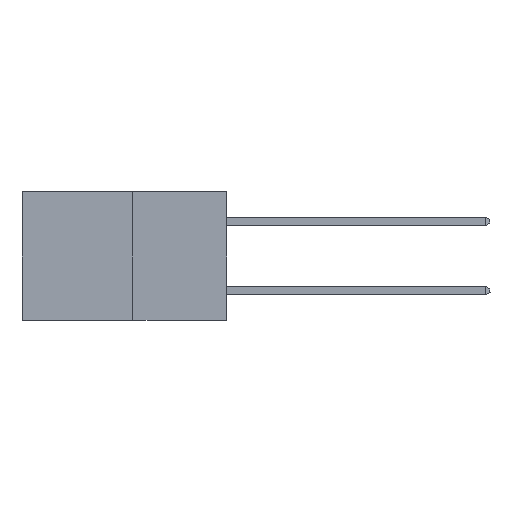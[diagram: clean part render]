
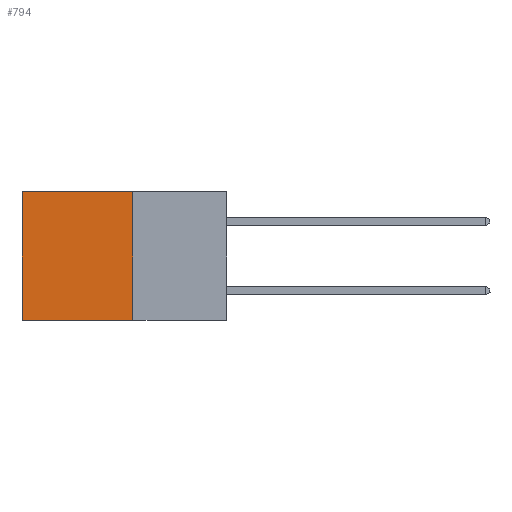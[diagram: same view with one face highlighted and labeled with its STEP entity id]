
A CAD part, left-side view. The second image highlights one B-rep face of the part: STEP entity #794.
In plain terms, the highlighted planar face has unit normal (-1, 0, 0).
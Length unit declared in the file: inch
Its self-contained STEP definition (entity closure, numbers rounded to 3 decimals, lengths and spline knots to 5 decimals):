
#794 = ADVANCED_FACE ( 'NONE', ( #16569 ), #21081, .F. ) ;
#3560 = CARTESIAN_POINT ( 'NONE',  ( 0.277, 0.27, 0. ) ) ;
#3947 = CARTESIAN_POINT ( 'NONE',  ( 0.277, 0.59, -0.37 ) ) ;
#4394 = EDGE_CURVE ( 'NONE', #24834, #8620, #6015, .T. ) ;
#4659 = DIRECTION ( 'NONE',  ( 1., 0., 0. ) ) ;
#5328 = VECTOR ( 'NONE', #27437, 39.37008 ) ;
#6015 = LINE ( 'NONE', #27498, #5328 ) ;
#6527 = CARTESIAN_POINT ( 'NONE',  ( 0.277, 0.27, -0.37 ) ) ;
#8620 = VERTEX_POINT ( 'NONE', #3947 ) ;
#8664 = DIRECTION ( 'NONE',  ( 0., 0., -1. ) ) ;
#8824 = EDGE_CURVE ( 'NONE', #20589, #24834, #24039, .T. ) ;
#9426 = CARTESIAN_POINT ( 'NONE',  ( 0.277, 0.59, -0.37 ) ) ;
#11299 = ORIENTED_EDGE ( 'NONE', *, *, #4394, .F. ) ;
#11416 = VECTOR ( 'NONE', #13048, 39.37008 ) ;
#12154 = EDGE_CURVE ( 'NONE', #25219, #8620, #25153, .T. ) ;
#12515 = CARTESIAN_POINT ( 'NONE',  ( 0.277, 0.59, 0. ) ) ;
#12981 = ORIENTED_EDGE ( 'NONE', *, *, #22750, .T. ) ;
#13013 = CARTESIAN_POINT ( 'NONE',  ( 0.277, 0.27, -0.37 ) ) ;
#13027 = DIRECTION ( 'NONE',  ( 0., 1., 0. ) ) ;
#13048 = DIRECTION ( 'NONE',  ( 0., 0., -1. ) ) ;
#15473 = LINE ( 'NONE', #17561, #28705 ) ;
#15789 = CARTESIAN_POINT ( 'NONE',  ( 0.277, 0.27, -0.37 ) ) ;
#16569 = FACE_OUTER_BOUND ( 'NONE', #19549, .T. ) ;
#17561 = CARTESIAN_POINT ( 'NONE',  ( 0.277, 0.27, 0. ) ) ;
#19256 = VECTOR ( 'NONE', #22971, 39.37008 ) ;
#19549 = EDGE_LOOP ( 'NONE', ( #25642, #11299, #28095, #12981 ) ) ;
#20589 = VERTEX_POINT ( 'NONE', #3560 ) ;
#21081 = PLANE ( 'NONE',  #27432 ) ;
#22750 = EDGE_CURVE ( 'NONE', #20589, #25219, #15473, .T. ) ;
#22971 = DIRECTION ( 'NONE',  ( 0., 0., -1. ) ) ;
#24039 = LINE ( 'NONE', #13013, #11416 ) ;
#24834 = VERTEX_POINT ( 'NONE', #15789 ) ;
#25153 = LINE ( 'NONE', #9426, #19256 ) ;
#25219 = VERTEX_POINT ( 'NONE', #12515 ) ;
#25642 = ORIENTED_EDGE ( 'NONE', *, *, #12154, .T. ) ;
#27432 = AXIS2_PLACEMENT_3D ( 'NONE', #6527, #4659, #8664 ) ;
#27437 = DIRECTION ( 'NONE',  ( 0., 1., 0. ) ) ;
#27498 = CARTESIAN_POINT ( 'NONE',  ( 0.277, 0.27, -0.37 ) ) ;
#28095 = ORIENTED_EDGE ( 'NONE', *, *, #8824, .F. ) ;
#28705 = VECTOR ( 'NONE', #13027, 39.37008 ) ;
